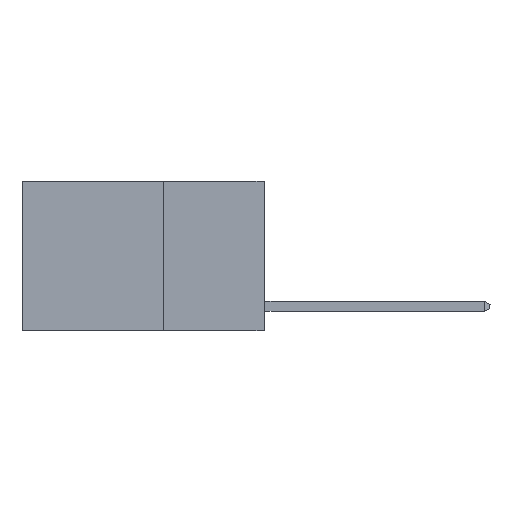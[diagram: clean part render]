
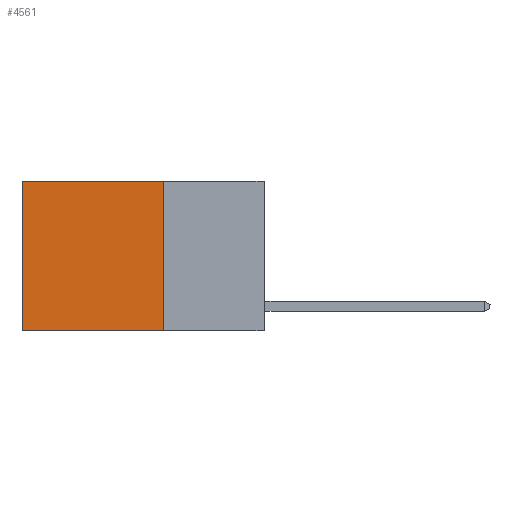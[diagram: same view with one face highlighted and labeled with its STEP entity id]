
A CAD part, left-side view. The second image highlights one B-rep face of the part: STEP entity #4561.
In plain terms, the highlighted planar face has unit normal (-1, 0, 0).
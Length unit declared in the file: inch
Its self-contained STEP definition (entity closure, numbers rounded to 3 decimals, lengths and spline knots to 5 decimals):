
#157 = DIRECTION ( 'NONE',  ( 0., 1., 0. ) ) ;
#785 = LINE ( 'NONE', #10937, #20924 ) ;
#1974 = CARTESIAN_POINT ( 'NONE',  ( 0.2625, 0.25, 0. ) ) ;
#2211 = CARTESIAN_POINT ( 'NONE',  ( 0.2625, 0.6, -0.37 ) ) ;
#2214 = EDGE_CURVE ( 'NONE', #7936, #10507, #3916, .T. ) ;
#3134 = ORIENTED_EDGE ( 'NONE', *, *, #2214, .F. ) ;
#3287 = EDGE_CURVE ( 'NONE', #10507, #3527, #7524, .T. ) ;
#3522 = DIRECTION ( 'NONE',  ( 0., 0., -1. ) ) ;
#3527 = VERTEX_POINT ( 'NONE', #2211 ) ;
#3916 = LINE ( 'NONE', #1974, #11500 ) ;
#4149 = VECTOR ( 'NONE', #6121, 39.37008 ) ;
#4397 = CARTESIAN_POINT ( 'NONE',  ( 0.2625, 0.25, 0. ) ) ;
#4467 = VERTEX_POINT ( 'NONE', #6158 ) ;
#4561 = ADVANCED_FACE ( 'NONE', ( #12492 ), #5292, .F. ) ;
#5292 = PLANE ( 'NONE',  #22034 ) ;
#5932 = LINE ( 'NONE', #15679, #22633 ) ;
#6121 = DIRECTION ( 'NONE',  ( 0., 1., 0. ) ) ;
#6158 = CARTESIAN_POINT ( 'NONE',  ( 0.2625, 0.6, 0. ) ) ;
#7524 = LINE ( 'NONE', #10029, #4149 ) ;
#7936 = VERTEX_POINT ( 'NONE', #4397 ) ;
#8375 = EDGE_LOOP ( 'NONE', ( #12535, #14646, #3134, #17309 ) ) ;
#9148 = CARTESIAN_POINT ( 'NONE',  ( 0.2625, 0.25, -0.37 ) ) ;
#9865 = EDGE_CURVE ( 'NONE', #4467, #3527, #5932, .T. ) ;
#10029 = CARTESIAN_POINT ( 'NONE',  ( 0.2625, 0.25, -0.37 ) ) ;
#10480 = EDGE_CURVE ( 'NONE', #7936, #4467, #785, .T. ) ;
#10507 = VERTEX_POINT ( 'NONE', #9148 ) ;
#10937 = CARTESIAN_POINT ( 'NONE',  ( 0.2625, 0.25, 0. ) ) ;
#11500 = VECTOR ( 'NONE', #16092, 39.37008 ) ;
#12469 = CARTESIAN_POINT ( 'NONE',  ( 0.2625, 0.25, 0. ) ) ;
#12492 = FACE_OUTER_BOUND ( 'NONE', #8375, .T. ) ;
#12535 = ORIENTED_EDGE ( 'NONE', *, *, #9865, .T. ) ;
#14255 = DIRECTION ( 'NONE',  ( 1., 0., 0. ) ) ;
#14646 = ORIENTED_EDGE ( 'NONE', *, *, #3287, .F. ) ;
#15679 = CARTESIAN_POINT ( 'NONE',  ( 0.2625, 0.6, 0. ) ) ;
#16092 = DIRECTION ( 'NONE',  ( 0., 0., -1. ) ) ;
#17309 = ORIENTED_EDGE ( 'NONE', *, *, #10480, .T. ) ;
#19317 = DIRECTION ( 'NONE',  ( 0., 0., -1. ) ) ;
#20924 = VECTOR ( 'NONE', #157, 39.37008 ) ;
#22034 = AXIS2_PLACEMENT_3D ( 'NONE', #12469, #14255, #3522 ) ;
#22633 = VECTOR ( 'NONE', #19317, 39.37008 ) ;
